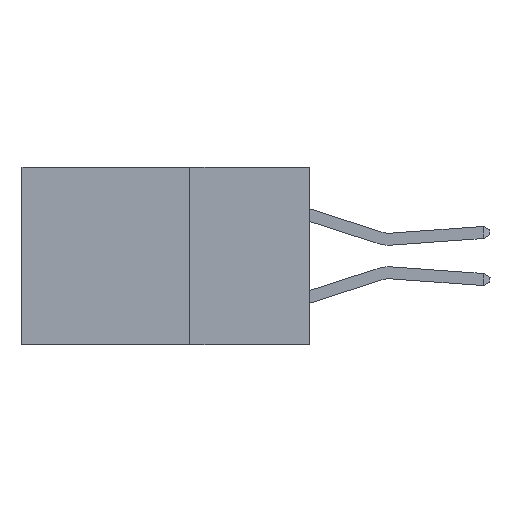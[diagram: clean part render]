
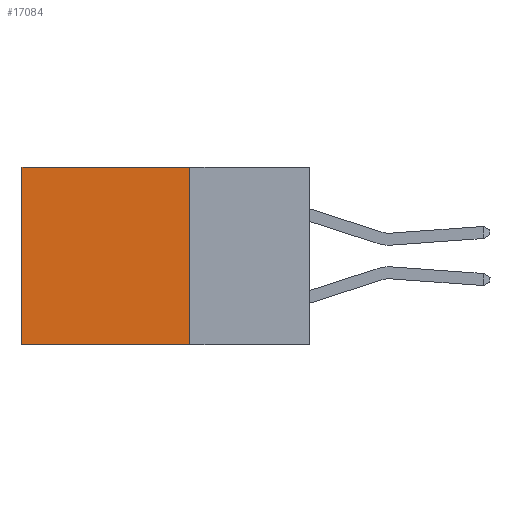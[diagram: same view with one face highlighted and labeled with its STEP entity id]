
A CAD part, left-side view. The second image highlights one B-rep face of the part: STEP entity #17084.
In plain terms, the highlighted planar face has unit normal (-1, 0, 0).
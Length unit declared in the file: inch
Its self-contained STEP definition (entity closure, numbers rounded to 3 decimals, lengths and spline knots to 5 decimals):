
#1202 = LINE ( 'NONE', #10524, #11965 ) ;
#2111 = EDGE_CURVE ( 'NONE', #5276, #9358, #16829, .T. ) ;
#2540 = CARTESIAN_POINT ( 'NONE',  ( 0.298, 0.25, 0. ) ) ;
#3674 = FACE_OUTER_BOUND ( 'NONE', #6582, .T. ) ;
#4289 = DIRECTION ( 'NONE',  ( 0., 0., -1. ) ) ;
#4688 = AXIS2_PLACEMENT_3D ( 'NONE', #27418, #17006, #4289 ) ;
#5276 = VERTEX_POINT ( 'NONE', #2540 ) ;
#5342 = DIRECTION ( 'NONE',  ( 0., 0., -1. ) ) ;
#5499 = EDGE_CURVE ( 'NONE', #9358, #6717, #16300, .T. ) ;
#6582 = EDGE_LOOP ( 'NONE', ( #10085, #11957, #7437, #15143 ) ) ;
#6600 = CARTESIAN_POINT ( 'NONE',  ( 0.298, 0.25, -0.37 ) ) ;
#6717 = VERTEX_POINT ( 'NONE', #12856 ) ;
#7437 = ORIENTED_EDGE ( 'NONE', *, *, #2111, .F. ) ;
#8390 = EDGE_CURVE ( 'NONE', #22531, #6717, #18600, .T. ) ;
#9358 = VERTEX_POINT ( 'NONE', #6600 ) ;
#10085 = ORIENTED_EDGE ( 'NONE', *, *, #8390, .T. ) ;
#10524 = CARTESIAN_POINT ( 'NONE',  ( 0.298, 0.25, 0. ) ) ;
#11231 = VECTOR ( 'NONE', #25731, 39.37008 ) ;
#11957 = ORIENTED_EDGE ( 'NONE', *, *, #5499, .F. ) ;
#11965 = VECTOR ( 'NONE', #12623, 39.37008 ) ;
#11993 = CARTESIAN_POINT ( 'NONE',  ( 0.298, 0.25, 0. ) ) ;
#12623 = DIRECTION ( 'NONE',  ( 0., 1., 0. ) ) ;
#12856 = CARTESIAN_POINT ( 'NONE',  ( 0.298, 0.6, -0.37 ) ) ;
#13819 = CARTESIAN_POINT ( 'NONE',  ( 0.298, 0.6, 0. ) ) ;
#14889 = PLANE ( 'NONE',  #4688 ) ;
#15143 = ORIENTED_EDGE ( 'NONE', *, *, #18218, .T. ) ;
#15150 = CARTESIAN_POINT ( 'NONE',  ( 0.298, 0.6, 0. ) ) ;
#16300 = LINE ( 'NONE', #22511, #20588 ) ;
#16829 = LINE ( 'NONE', #11993, #11231 ) ;
#17006 = DIRECTION ( 'NONE',  ( 1., 0., 0. ) ) ;
#17084 = ADVANCED_FACE ( 'NONE', ( #3674 ), #14889, .F. ) ;
#18218 = EDGE_CURVE ( 'NONE', #5276, #22531, #1202, .T. ) ;
#18600 = LINE ( 'NONE', #13819, #23516 ) ;
#20588 = VECTOR ( 'NONE', #22189, 39.37008 ) ;
#22189 = DIRECTION ( 'NONE',  ( 0., 1., 0. ) ) ;
#22511 = CARTESIAN_POINT ( 'NONE',  ( 0.298, 0.25, -0.37 ) ) ;
#22531 = VERTEX_POINT ( 'NONE', #15150 ) ;
#23516 = VECTOR ( 'NONE', #5342, 39.37008 ) ;
#25731 = DIRECTION ( 'NONE',  ( 0., 0., -1. ) ) ;
#27418 = CARTESIAN_POINT ( 'NONE',  ( 0.298, 0.25, 0. ) ) ;
